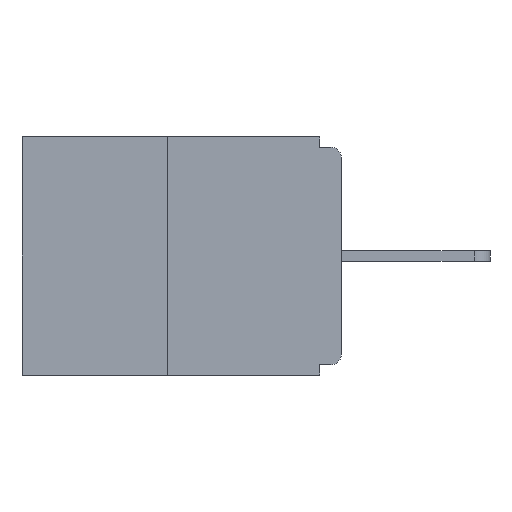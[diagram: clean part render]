
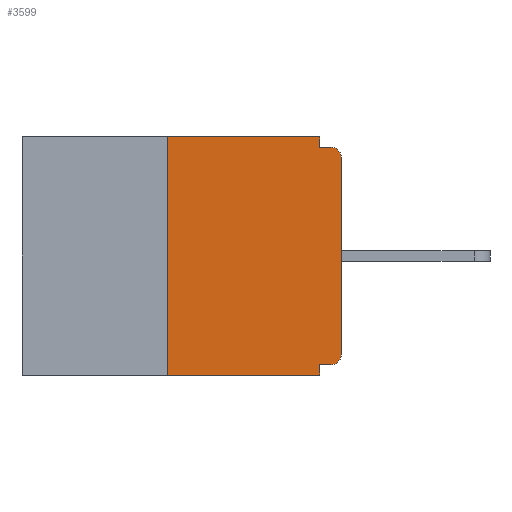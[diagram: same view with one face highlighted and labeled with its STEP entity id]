
A CAD part, left-side view. The second image highlights one B-rep face of the part: STEP entity #3599.
In plain terms, the highlighted planar face has unit normal (-1, 0, 0).
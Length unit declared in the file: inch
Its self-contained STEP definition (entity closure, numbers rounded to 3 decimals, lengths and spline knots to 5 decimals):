
#83 = CARTESIAN_POINT ( 'NONE',  ( 0., 0., -0.313 ) ) ;
#175 = ORIENTED_EDGE ( 'NONE', *, *, #2561, .T. ) ;
#522 = LINE ( 'NONE', #11091, #13209 ) ;
#542 = VERTEX_POINT ( 'NONE', #3604 ) ;
#545 = VECTOR ( 'NONE', #3067, 39.37008 ) ;
#868 = DIRECTION ( 'NONE',  ( 0., 0., 1. ) ) ;
#1093 = LINE ( 'NONE', #5681, #13351 ) ;
#1380 = ORIENTED_EDGE ( 'NONE', *, *, #12725, .T. ) ;
#1450 = VERTEX_POINT ( 'NONE', #9717 ) ;
#1559 = AXIS2_PLACEMENT_3D ( 'NONE', #12513, #5509, #13683 ) ;
#1659 = CARTESIAN_POINT ( 'NONE',  ( 0., 0.46, 0. ) ) ;
#1718 = EDGE_CURVE ( 'NONE', #7683, #13475, #3859, .T. ) ;
#1728 = CARTESIAN_POINT ( 'NONE',  ( 0., 0.031, 0. ) ) ;
#1781 = ORIENTED_EDGE ( 'NONE', *, *, #7563, .T. ) ;
#2193 = ORIENTED_EDGE ( 'NONE', *, *, #3430, .F. ) ;
#2283 = CARTESIAN_POINT ( 'NONE',  ( 0., 0., 0. ) ) ;
#2421 = VECTOR ( 'NONE', #14612, 39.37008 ) ;
#2561 = EDGE_CURVE ( 'NONE', #4140, #13475, #522, .T. ) ;
#2666 = VERTEX_POINT ( 'NONE', #6117 ) ;
#2676 = LINE ( 'NONE', #13697, #11723 ) ;
#2790 = CARTESIAN_POINT ( 'NONE',  ( 0., 0.031, -0.328 ) ) ;
#3067 = DIRECTION ( 'NONE',  ( 0., 0., -1. ) ) ;
#3126 = ORIENTED_EDGE ( 'NONE', *, *, #4155, .F. ) ;
#3199 = VECTOR ( 'NONE', #3488, 39.37008 ) ;
#3430 = EDGE_CURVE ( 'NONE', #542, #14132, #3641, .T. ) ;
#3488 = DIRECTION ( 'NONE',  ( 0., 0., 1. ) ) ;
#3599 = ADVANCED_FACE ( 'NONE', ( #7367 ), #12576, .F. ) ;
#3604 = CARTESIAN_POINT ( 'NONE',  ( 0., 0.031, 0. ) ) ;
#3641 = LINE ( 'NONE', #1728, #9588 ) ;
#3859 = LINE ( 'NONE', #12137, #545 ) ;
#3872 = ORIENTED_EDGE ( 'NONE', *, *, #4069, .F. ) ;
#3915 = CARTESIAN_POINT ( 'NONE',  ( 0., 0.015, -0.328 ) ) ;
#4069 = EDGE_CURVE ( 'NONE', #10626, #7683, #2676, .T. ) ;
#4140 = VERTEX_POINT ( 'NONE', #8072 ) ;
#4155 = EDGE_CURVE ( 'NONE', #4140, #15149, #1093, .T. ) ;
#4428 = VERTEX_POINT ( 'NONE', #83 ) ;
#4442 = DIRECTION ( 'NONE',  ( 0., -1., 0. ) ) ;
#4522 = DIRECTION ( 'NONE',  ( 0., 0., -1. ) ) ;
#4765 = AXIS2_PLACEMENT_3D ( 'NONE', #7285, #12381, #8487 ) ;
#5489 = DIRECTION ( 'NONE',  ( 1., 0., 0. ) ) ;
#5509 = DIRECTION ( 'NONE',  ( -1., 0., 0. ) ) ;
#5681 = CARTESIAN_POINT ( 'NONE',  ( 0., 0.25, 0. ) ) ;
#6078 = VECTOR ( 'NONE', #4442, 39.37008 ) ;
#6117 = CARTESIAN_POINT ( 'NONE',  ( 0., 0.015, -0.015 ) ) ;
#6120 = DIRECTION ( 'NONE',  ( 0., 0., -1. ) ) ;
#6209 = CARTESIAN_POINT ( 'NONE',  ( 0., 0.46, 0. ) ) ;
#6269 = EDGE_CURVE ( 'NONE', #15149, #542, #8745, .T. ) ;
#6691 = CARTESIAN_POINT ( 'NONE',  ( 0., 0.25, 0. ) ) ;
#7285 = CARTESIAN_POINT ( 'NONE',  ( 0., 0.015, -0.03 ) ) ;
#7367 = FACE_OUTER_BOUND ( 'NONE', #12292, .T. ) ;
#7563 = EDGE_CURVE ( 'NONE', #1450, #2666, #12001, .T. ) ;
#7683 = VERTEX_POINT ( 'NONE', #2790 ) ;
#8072 = CARTESIAN_POINT ( 'NONE',  ( 0., 0.25, -0.343 ) ) ;
#8168 = ORIENTED_EDGE ( 'NONE', *, *, #13789, .F. ) ;
#8487 = DIRECTION ( 'NONE',  ( 0., 0., -1. ) ) ;
#8745 = LINE ( 'NONE', #1659, #2421 ) ;
#9222 = LINE ( 'NONE', #10337, #6078 ) ;
#9509 = LINE ( 'NONE', #2283, #3199 ) ;
#9588 = VECTOR ( 'NONE', #6120, 39.37008 ) ;
#9687 = AXIS2_PLACEMENT_3D ( 'NONE', #6209, #5489, #4522 ) ;
#9717 = CARTESIAN_POINT ( 'NONE',  ( 0., 0., -0.03 ) ) ;
#9805 = ORIENTED_EDGE ( 'NONE', *, *, #1718, .F. ) ;
#10207 = DIRECTION ( 'NONE',  ( 0., 1., 0. ) ) ;
#10337 = CARTESIAN_POINT ( 'NONE',  ( 0., 0., -0.015 ) ) ;
#10533 = ORIENTED_EDGE ( 'NONE', *, *, #11456, .T. ) ;
#10626 = VERTEX_POINT ( 'NONE', #3915 ) ;
#11086 = DIRECTION ( 'NONE',  ( 0., -1., 0. ) ) ;
#11091 = CARTESIAN_POINT ( 'NONE',  ( 0., 0.46, -0.343 ) ) ;
#11456 = EDGE_CURVE ( 'NONE', #10626, #4428, #14622, .T. ) ;
#11723 = VECTOR ( 'NONE', #10207, 39.37008 ) ;
#12001 = CIRCLE ( 'NONE', #4765, 0.015 ) ;
#12137 = CARTESIAN_POINT ( 'NONE',  ( 0., 0.031, -0.343 ) ) ;
#12292 = EDGE_LOOP ( 'NONE', ( #14877, #3126, #175, #9805, #3872, #10533, #1380, #1781, #8168, #2193 ) ) ;
#12381 = DIRECTION ( 'NONE',  ( -1., 0., 0. ) ) ;
#12513 = CARTESIAN_POINT ( 'NONE',  ( 0., 0.015, -0.313 ) ) ;
#12576 = PLANE ( 'NONE',  #9687 ) ;
#12725 = EDGE_CURVE ( 'NONE', #4428, #1450, #9509, .T. ) ;
#13209 = VECTOR ( 'NONE', #11086, 39.37008 ) ;
#13351 = VECTOR ( 'NONE', #868, 39.37008 ) ;
#13475 = VERTEX_POINT ( 'NONE', #14497 ) ;
#13683 = DIRECTION ( 'NONE',  ( 0., 0., -1. ) ) ;
#13697 = CARTESIAN_POINT ( 'NONE',  ( 0., 0., -0.328 ) ) ;
#13789 = EDGE_CURVE ( 'NONE', #14132, #2666, #9222, .T. ) ;
#14132 = VERTEX_POINT ( 'NONE', #14330 ) ;
#14330 = CARTESIAN_POINT ( 'NONE',  ( 0., 0.031, -0.015 ) ) ;
#14497 = CARTESIAN_POINT ( 'NONE',  ( 0., 0.031, -0.343 ) ) ;
#14612 = DIRECTION ( 'NONE',  ( 0., -1., 0. ) ) ;
#14622 = CIRCLE ( 'NONE', #1559, 0.015 ) ;
#14877 = ORIENTED_EDGE ( 'NONE', *, *, #6269, .F. ) ;
#15149 = VERTEX_POINT ( 'NONE', #6691 ) ;
